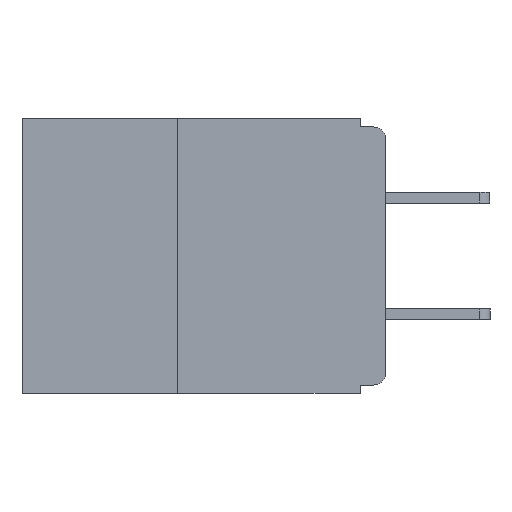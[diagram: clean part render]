
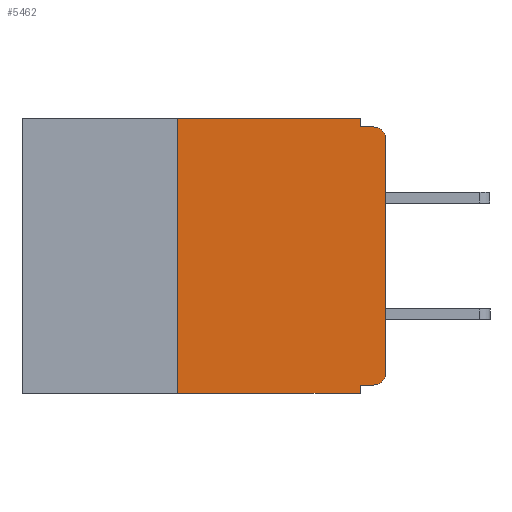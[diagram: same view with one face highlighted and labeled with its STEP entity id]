
A CAD part, left-side view. The second image highlights one B-rep face of the part: STEP entity #5462.
In plain terms, the highlighted planar face has unit normal (-1, 0, 0).
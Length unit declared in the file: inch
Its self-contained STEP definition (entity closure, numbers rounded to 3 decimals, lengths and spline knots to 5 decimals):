
#46 = VERTEX_POINT ( 'NONE', #2872 ) ;
#91 = DIRECTION ( 'NONE',  ( 0., 0., -1. ) ) ;
#296 = CARTESIAN_POINT ( 'NONE',  ( 0., 0.031, 0. ) ) ;
#511 = CARTESIAN_POINT ( 'NONE',  ( 0., 0., 0. ) ) ;
#1415 = DIRECTION ( 'NONE',  ( -1., 0., 0. ) ) ;
#1563 = CIRCLE ( 'NONE', #6459, 0.015 ) ;
#1576 = DIRECTION ( 'NONE',  ( 0., 0., 1. ) ) ;
#1659 = CARTESIAN_POINT ( 'NONE',  ( 0., 0.25, -0.33 ) ) ;
#1750 = EDGE_CURVE ( 'NONE', #12304, #10203, #14235, .T. ) ;
#2026 = EDGE_CURVE ( 'NONE', #46, #11183, #5276, .T. ) ;
#2138 = VECTOR ( 'NONE', #1576, 39.37008 ) ;
#2140 = EDGE_CURVE ( 'NONE', #46, #7470, #12439, .T. ) ;
#2223 = CARTESIAN_POINT ( 'NONE',  ( 0., 0.031, -0.32 ) ) ;
#2872 = CARTESIAN_POINT ( 'NONE',  ( 0., 0.25, -0.33 ) ) ;
#2982 = CARTESIAN_POINT ( 'NONE',  ( 0., 0.031, 0. ) ) ;
#3087 = LINE ( 'NONE', #4695, #8887 ) ;
#3149 = CARTESIAN_POINT ( 'NONE',  ( 0., 0., -0.025 ) ) ;
#3271 = DIRECTION ( 'NONE',  ( 0., -1., 0. ) ) ;
#3363 = CARTESIAN_POINT ( 'NONE',  ( 0., 0.015, -0.32 ) ) ;
#3482 = CARTESIAN_POINT ( 'NONE',  ( 0., 0.25, 0. ) ) ;
#4259 = EDGE_CURVE ( 'NONE', #8592, #8579, #9627, .T. ) ;
#4372 = CARTESIAN_POINT ( 'NONE',  ( 0., 0.031, -0.33 ) ) ;
#4588 = LINE ( 'NONE', #6440, #7301 ) ;
#4695 = CARTESIAN_POINT ( 'NONE',  ( 0., 0., -0.32 ) ) ;
#5095 = CARTESIAN_POINT ( 'NONE',  ( 0., 0., -0.01 ) ) ;
#5116 = DIRECTION ( 'NONE',  ( 0., -1., 0. ) ) ;
#5276 = LINE ( 'NONE', #1659, #2138 ) ;
#5329 = DIRECTION ( 'NONE',  ( 0., 0., -1. ) ) ;
#5451 = ORIENTED_EDGE ( 'NONE', *, *, #4259, .T. ) ;
#5462 = ADVANCED_FACE ( 'NONE', ( #14418 ), #8591, .F. ) ;
#5765 = CARTESIAN_POINT ( 'NONE',  ( 0., 0.437, 0. ) ) ;
#5887 = CARTESIAN_POINT ( 'NONE',  ( 0., 0.015, -0.025 ) ) ;
#5950 = ORIENTED_EDGE ( 'NONE', *, *, #14484, .T. ) ;
#6059 = ORIENTED_EDGE ( 'NONE', *, *, #1750, .F. ) ;
#6106 = EDGE_CURVE ( 'NONE', #12063, #11144, #3087, .T. ) ;
#6236 = EDGE_CURVE ( 'NONE', #12063, #8592, #1563, .T. ) ;
#6290 = EDGE_LOOP ( 'NONE', ( #5451, #5950, #6059, #6392, #6452, #7248, #7407, #8000, #8932, #9943 ) ) ;
#6296 = CARTESIAN_POINT ( 'NONE',  ( 0., 0.031, -0.01 ) ) ;
#6392 = ORIENTED_EDGE ( 'NONE', *, *, #13030, .F. ) ;
#6440 = CARTESIAN_POINT ( 'NONE',  ( 0., 0.437, 0. ) ) ;
#6452 = ORIENTED_EDGE ( 'NONE', *, *, #9829, .F. ) ;
#6459 = AXIS2_PLACEMENT_3D ( 'NONE', #9947, #1415, #91 ) ;
#6480 = VECTOR ( 'NONE', #5329, 39.37008 ) ;
#6493 = VERTEX_POINT ( 'NONE', #296 ) ;
#6519 = VECTOR ( 'NONE', #3271, 39.37008 ) ;
#6558 = AXIS2_PLACEMENT_3D ( 'NONE', #5765, #13941, #13123 ) ;
#6584 = VECTOR ( 'NONE', #8400, 39.37008 ) ;
#6689 = CARTESIAN_POINT ( 'NONE',  ( 0., 0., -0.305 ) ) ;
#7026 = DIRECTION ( 'NONE',  ( 0., 0., -1. ) ) ;
#7248 = ORIENTED_EDGE ( 'NONE', *, *, #2026, .F. ) ;
#7301 = VECTOR ( 'NONE', #12003, 39.37008 ) ;
#7407 = ORIENTED_EDGE ( 'NONE', *, *, #2140, .T. ) ;
#7470 = VERTEX_POINT ( 'NONE', #13426 ) ;
#8000 = ORIENTED_EDGE ( 'NONE', *, *, #11677, .F. ) ;
#8318 = CARTESIAN_POINT ( 'NONE',  ( 0., 0.015, -0.01 ) ) ;
#8400 = DIRECTION ( 'NONE',  ( 0., 0., 1. ) ) ;
#8445 = AXIS2_PLACEMENT_3D ( 'NONE', #5887, #13611, #7026 ) ;
#8534 = VECTOR ( 'NONE', #5116, 39.37008 ) ;
#8579 = VERTEX_POINT ( 'NONE', #3149 ) ;
#8591 = PLANE ( 'NONE',  #6558 ) ;
#8592 = VERTEX_POINT ( 'NONE', #6689 ) ;
#8887 = VECTOR ( 'NONE', #10462, 39.37008 ) ;
#8932 = ORIENTED_EDGE ( 'NONE', *, *, #6106, .F. ) ;
#9534 = LINE ( 'NONE', #2982, #6480 ) ;
#9627 = LINE ( 'NONE', #511, #6584 ) ;
#9829 = EDGE_CURVE ( 'NONE', #11183, #6493, #4588, .T. ) ;
#9943 = ORIENTED_EDGE ( 'NONE', *, *, #6236, .T. ) ;
#9947 = CARTESIAN_POINT ( 'NONE',  ( 0., 0.015, -0.305 ) ) ;
#10203 = VERTEX_POINT ( 'NONE', #8318 ) ;
#10462 = DIRECTION ( 'NONE',  ( 0., 1., 0. ) ) ;
#10759 = LINE ( 'NONE', #4372, #13583 ) ;
#11144 = VERTEX_POINT ( 'NONE', #2223 ) ;
#11151 = DIRECTION ( 'NONE',  ( 0., 0., -1. ) ) ;
#11183 = VERTEX_POINT ( 'NONE', #3482 ) ;
#11571 = CARTESIAN_POINT ( 'NONE',  ( 0., 0.437, -0.33 ) ) ;
#11677 = EDGE_CURVE ( 'NONE', #11144, #7470, #10759, .T. ) ;
#12003 = DIRECTION ( 'NONE',  ( 0., -1., 0. ) ) ;
#12063 = VERTEX_POINT ( 'NONE', #3363 ) ;
#12304 = VERTEX_POINT ( 'NONE', #6296 ) ;
#12439 = LINE ( 'NONE', #11571, #6519 ) ;
#13030 = EDGE_CURVE ( 'NONE', #6493, #12304, #9534, .T. ) ;
#13123 = DIRECTION ( 'NONE',  ( 0., 0., -1. ) ) ;
#13426 = CARTESIAN_POINT ( 'NONE',  ( 0., 0.031, -0.33 ) ) ;
#13583 = VECTOR ( 'NONE', #11151, 39.37008 ) ;
#13611 = DIRECTION ( 'NONE',  ( -1., 0., 0. ) ) ;
#13941 = DIRECTION ( 'NONE',  ( 1., 0., 0. ) ) ;
#14004 = CIRCLE ( 'NONE', #8445, 0.015 ) ;
#14235 = LINE ( 'NONE', #5095, #8534 ) ;
#14418 = FACE_OUTER_BOUND ( 'NONE', #6290, .T. ) ;
#14484 = EDGE_CURVE ( 'NONE', #8579, #10203, #14004, .T. ) ;
